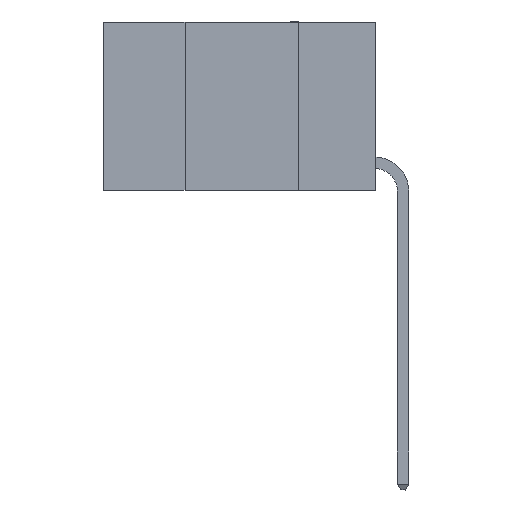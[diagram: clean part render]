
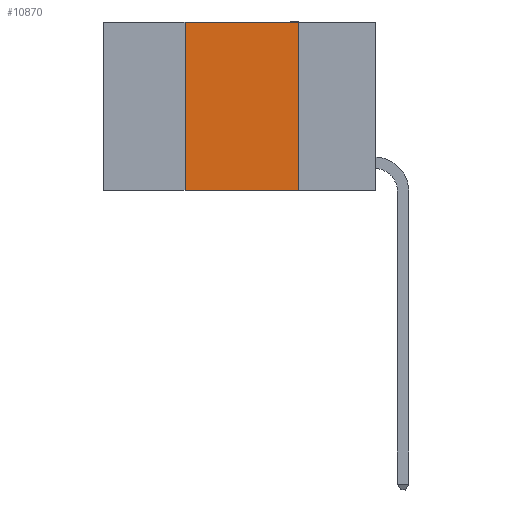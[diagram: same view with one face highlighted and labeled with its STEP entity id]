
A CAD part, left-side view. The second image highlights one B-rep face of the part: STEP entity #10870.
In plain terms, the highlighted planar face has unit normal (-1, 0, 0).
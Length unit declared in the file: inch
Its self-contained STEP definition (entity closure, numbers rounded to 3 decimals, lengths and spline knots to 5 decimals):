
#1365 = CARTESIAN_POINT ( 'NONE',  ( 0., 0.42, 0. ) ) ;
#2616 = EDGE_CURVE ( 'NONE', #13398, #7539, #21179, .T. ) ;
#2834 = VECTOR ( 'NONE', #7235, 39.37008 ) ;
#3456 = EDGE_CURVE ( 'NONE', #4167, #6967, #13506, .T. ) ;
#3742 = VECTOR ( 'NONE', #16183, 39.37008 ) ;
#4167 = VERTEX_POINT ( 'NONE', #16361 ) ;
#5243 = ORIENTED_EDGE ( 'NONE', *, *, #11302, .F. ) ;
#5835 = CARTESIAN_POINT ( 'NONE',  ( 0., 0.42, 0. ) ) ;
#6004 = VECTOR ( 'NONE', #19280, 39.37008 ) ;
#6328 = FACE_OUTER_BOUND ( 'NONE', #13885, .T. ) ;
#6430 = PLANE ( 'NONE',  #10126 ) ;
#6581 = EDGE_CURVE ( 'NONE', #7539, #6967, #15733, .T. ) ;
#6967 = VERTEX_POINT ( 'NONE', #11695 ) ;
#7235 = DIRECTION ( 'NONE',  ( 0., -1., 0. ) ) ;
#7539 = VERTEX_POINT ( 'NONE', #13205 ) ;
#8327 = VECTOR ( 'NONE', #18888, 39.37008 ) ;
#8604 = ORIENTED_EDGE ( 'NONE', *, *, #3456, .T. ) ;
#9818 = DIRECTION ( 'NONE',  ( 1., 0., 0. ) ) ;
#10126 = AXIS2_PLACEMENT_3D ( 'NONE', #20279, #9818, #21989 ) ;
#10870 = ADVANCED_FACE ( 'NONE', ( #6328 ), #6430, .F. ) ;
#10950 = CARTESIAN_POINT ( 'NONE',  ( 0., 0.6, 0. ) ) ;
#11302 = EDGE_CURVE ( 'NONE', #4167, #13398, #12292, .T. ) ;
#11695 = CARTESIAN_POINT ( 'NONE',  ( 0., 0.17, -0.37 ) ) ;
#12292 = LINE ( 'NONE', #5835, #3742 ) ;
#13205 = CARTESIAN_POINT ( 'NONE',  ( 0., 0.17, 0. ) ) ;
#13398 = VERTEX_POINT ( 'NONE', #1365 ) ;
#13506 = LINE ( 'NONE', #16664, #8327 ) ;
#13885 = EDGE_LOOP ( 'NONE', ( #19821, #21957, #5243, #8604 ) ) ;
#15733 = LINE ( 'NONE', #15788, #6004 ) ;
#15788 = CARTESIAN_POINT ( 'NONE',  ( 0., 0.17, 0. ) ) ;
#16183 = DIRECTION ( 'NONE',  ( 0., 0., 1. ) ) ;
#16361 = CARTESIAN_POINT ( 'NONE',  ( 0., 0.42, -0.37 ) ) ;
#16664 = CARTESIAN_POINT ( 'NONE',  ( 0., 0.6, -0.37 ) ) ;
#18888 = DIRECTION ( 'NONE',  ( 0., -1., 0. ) ) ;
#19280 = DIRECTION ( 'NONE',  ( 0., 0., -1. ) ) ;
#19821 = ORIENTED_EDGE ( 'NONE', *, *, #6581, .F. ) ;
#20279 = CARTESIAN_POINT ( 'NONE',  ( 0., 0.6, 0. ) ) ;
#21179 = LINE ( 'NONE', #10950, #2834 ) ;
#21957 = ORIENTED_EDGE ( 'NONE', *, *, #2616, .F. ) ;
#21989 = DIRECTION ( 'NONE',  ( 0., 0., -1. ) ) ;
